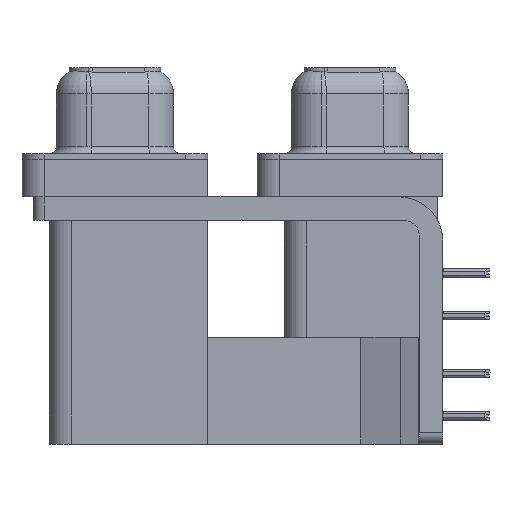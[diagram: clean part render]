
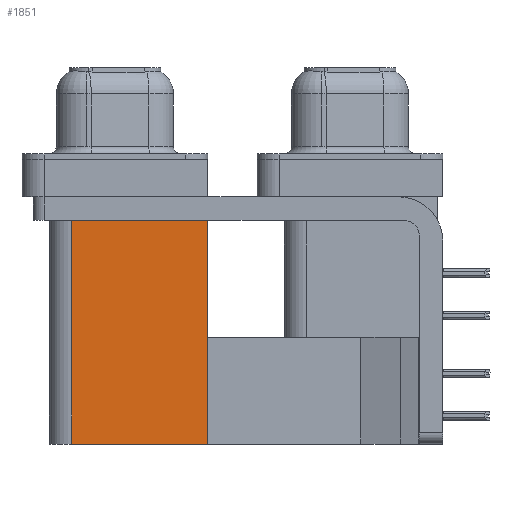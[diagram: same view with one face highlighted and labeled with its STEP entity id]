
A CAD part, left-side view. The second image highlights one B-rep face of the part: STEP entity #1851.
In plain terms, the highlighted planar face has unit normal (-1, 0, 0).
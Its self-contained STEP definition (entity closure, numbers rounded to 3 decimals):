
#806 = LINE ( 'NONE', #13028, #36342 ) ;
#1092 = VECTOR ( 'NONE', #13150, 1000. ) ;
#1442 = ORIENTED_EDGE ( 'NONE', *, *, #24823, .T. ) ;
#1851 = ADVANCED_FACE ( 'NONE', ( #36513 ), #20902, .F. ) ;
#2290 = DIRECTION ( 'NONE',  ( 0., 1., 0. ) ) ;
#4242 = VERTEX_POINT ( 'NONE', #5746 ) ;
#5682 = DIRECTION ( 'NONE',  ( 1., 0., 0. ) ) ;
#5746 = CARTESIAN_POINT ( 'NONE',  ( 3.79, 9.6, -19.2 ) ) ;
#5882 = ORIENTED_EDGE ( 'NONE', *, *, #39214, .F. ) ;
#5956 = DIRECTION ( 'NONE',  ( 0., 1., 0. ) ) ;
#6593 = CARTESIAN_POINT ( 'NONE',  ( 3.79, 9.6, -19.2 ) ) ;
#9199 = DIRECTION ( 'NONE',  ( 0., 1., 0. ) ) ;
#10632 = CARTESIAN_POINT ( 'NONE',  ( 3.79, 18.8, -2.5 ) ) ;
#12609 = EDGE_LOOP ( 'NONE', ( #32240, #34174, #5882, #1442 ) ) ;
#13028 = CARTESIAN_POINT ( 'NONE',  ( 3.79, 18.8, -19.2 ) ) ;
#13150 = DIRECTION ( 'NONE',  ( 0., 0., 1. ) ) ;
#13223 = DIRECTION ( 'NONE',  ( 0., 0., 1. ) ) ;
#14470 = CARTESIAN_POINT ( 'NONE',  ( 3.79, 18.8, -19.2 ) ) ;
#16444 = VECTOR ( 'NONE', #5956, 1000. ) ;
#18376 = LINE ( 'NONE', #34574, #1092 ) ;
#19690 = AXIS2_PLACEMENT_3D ( 'NONE', #23715, #5682, #2290 ) ;
#20902 = PLANE ( 'NONE',  #19690 ) ;
#22271 = VECTOR ( 'NONE', #9199, 1000. ) ;
#23715 = CARTESIAN_POINT ( 'NONE',  ( 3.79, 9.6, -19.2 ) ) ;
#24168 = LINE ( 'NONE', #27568, #16444 ) ;
#24823 = EDGE_CURVE ( 'NONE', #4242, #35323, #18376, .T. ) ;
#26865 = EDGE_CURVE ( 'NONE', #35323, #27377, #24168, .T. ) ;
#27377 = VERTEX_POINT ( 'NONE', #10632 ) ;
#27568 = CARTESIAN_POINT ( 'NONE',  ( 3.79, 9.6, -2.5 ) ) ;
#28803 = EDGE_CURVE ( 'NONE', #33446, #27377, #806, .T. ) ;
#32240 = ORIENTED_EDGE ( 'NONE', *, *, #26865, .T. ) ;
#33446 = VERTEX_POINT ( 'NONE', #14470 ) ;
#33634 = LINE ( 'NONE', #6593, #22271 ) ;
#34174 = ORIENTED_EDGE ( 'NONE', *, *, #28803, .F. ) ;
#34574 = CARTESIAN_POINT ( 'NONE',  ( 3.79, 9.6, -19.2 ) ) ;
#35323 = VERTEX_POINT ( 'NONE', #37221 ) ;
#36342 = VECTOR ( 'NONE', #13223, 1000. ) ;
#36513 = FACE_OUTER_BOUND ( 'NONE', #12609, .T. ) ;
#37221 = CARTESIAN_POINT ( 'NONE',  ( 3.79, 9.6, -2.5 ) ) ;
#39214 = EDGE_CURVE ( 'NONE', #4242, #33446, #33634, .T. ) ;
